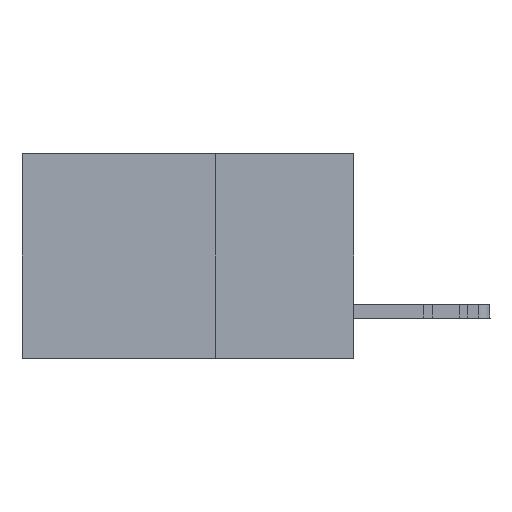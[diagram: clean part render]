
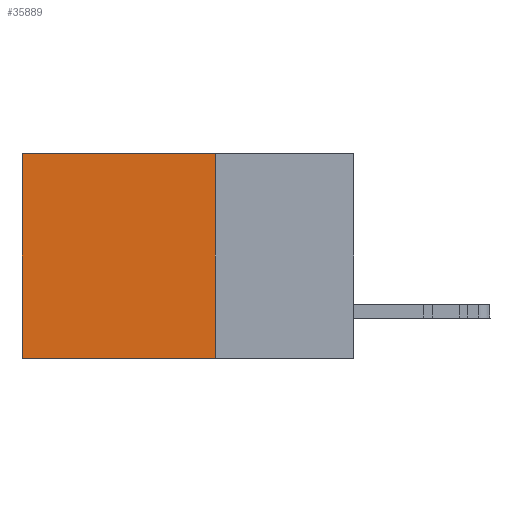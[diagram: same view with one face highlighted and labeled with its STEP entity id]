
A CAD part, left-side view. The second image highlights one B-rep face of the part: STEP entity #35889.
In plain terms, the highlighted planar face has unit normal (-1, 0, 0).
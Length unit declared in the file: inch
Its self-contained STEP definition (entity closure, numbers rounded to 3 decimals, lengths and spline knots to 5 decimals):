
#1211 = CARTESIAN_POINT ( 'NONE',  ( 0.2875, 0.25, -0.37 ) ) ;
#1320 = CARTESIAN_POINT ( 'NONE',  ( 0.2875, 0.25, 0. ) ) ;
#1692 = VERTEX_POINT ( 'NONE', #1211 ) ;
#3716 = EDGE_CURVE ( 'NONE', #12029, #30809, #34647, .T. ) ;
#4110 = EDGE_CURVE ( 'NONE', #1692, #30809, #31707, .T. ) ;
#4608 = CARTESIAN_POINT ( 'NONE',  ( 0.2875, 0.6, -0.37 ) ) ;
#4877 = CARTESIAN_POINT ( 'NONE',  ( 0.2875, 0.6, 0. ) ) ;
#5825 = DIRECTION ( 'NONE',  ( 0., 0., -1. ) ) ;
#6005 = CARTESIAN_POINT ( 'NONE',  ( 0.2875, 0.6, 0. ) ) ;
#7343 = CARTESIAN_POINT ( 'NONE',  ( 0.2875, 0.25, 0. ) ) ;
#8845 = VERTEX_POINT ( 'NONE', #30743 ) ;
#10354 = VECTOR ( 'NONE', #36772, 39.37008 ) ;
#12029 = VERTEX_POINT ( 'NONE', #6005 ) ;
#15409 = VECTOR ( 'NONE', #5825, 39.37008 ) ;
#17738 = CARTESIAN_POINT ( 'NONE',  ( 0.2875, 0.25, 0. ) ) ;
#19456 = VECTOR ( 'NONE', #48132, 39.37008 ) ;
#19545 = ORIENTED_EDGE ( 'NONE', *, *, #25764, .T. ) ;
#21214 = ORIENTED_EDGE ( 'NONE', *, *, #29114, .F. ) ;
#22562 = LINE ( 'NONE', #7343, #10354 ) ;
#25764 = EDGE_CURVE ( 'NONE', #8845, #12029, #22562, .T. ) ;
#29114 = EDGE_CURVE ( 'NONE', #8845, #1692, #39967, .T. ) ;
#30743 = CARTESIAN_POINT ( 'NONE',  ( 0.2875, 0.25, 0. ) ) ;
#30809 = VERTEX_POINT ( 'NONE', #4608 ) ;
#31171 = AXIS2_PLACEMENT_3D ( 'NONE', #17738, #36896, #40615 ) ;
#31223 = EDGE_LOOP ( 'NONE', ( #38007, #36786, #21214, #19545 ) ) ;
#31707 = LINE ( 'NONE', #47485, #19456 ) ;
#34647 = LINE ( 'NONE', #4877, #45687 ) ;
#35889 = ADVANCED_FACE ( 'NONE', ( #36735 ), #47321, .F. ) ;
#36735 = FACE_OUTER_BOUND ( 'NONE', #31223, .T. ) ;
#36772 = DIRECTION ( 'NONE',  ( 0., 1., 0. ) ) ;
#36786 = ORIENTED_EDGE ( 'NONE', *, *, #4110, .F. ) ;
#36896 = DIRECTION ( 'NONE',  ( 1., 0., 0. ) ) ;
#38007 = ORIENTED_EDGE ( 'NONE', *, *, #3716, .T. ) ;
#39967 = LINE ( 'NONE', #1320, #15409 ) ;
#40615 = DIRECTION ( 'NONE',  ( 0., 0., -1. ) ) ;
#45687 = VECTOR ( 'NONE', #46354, 39.37008 ) ;
#46354 = DIRECTION ( 'NONE',  ( 0., 0., -1. ) ) ;
#47321 = PLANE ( 'NONE',  #31171 ) ;
#47485 = CARTESIAN_POINT ( 'NONE',  ( 0.2875, 0.25, -0.37 ) ) ;
#48132 = DIRECTION ( 'NONE',  ( 0., 1., 0. ) ) ;
